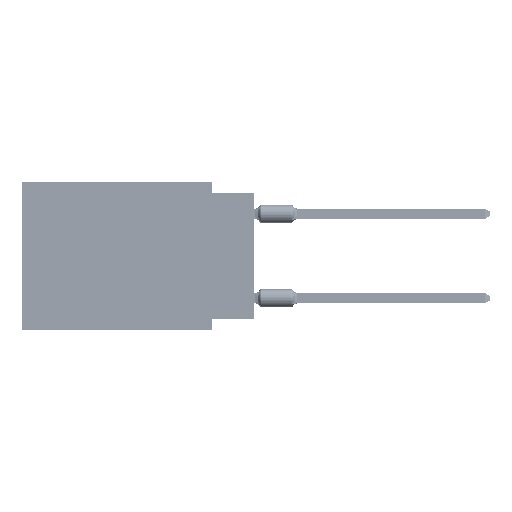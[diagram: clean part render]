
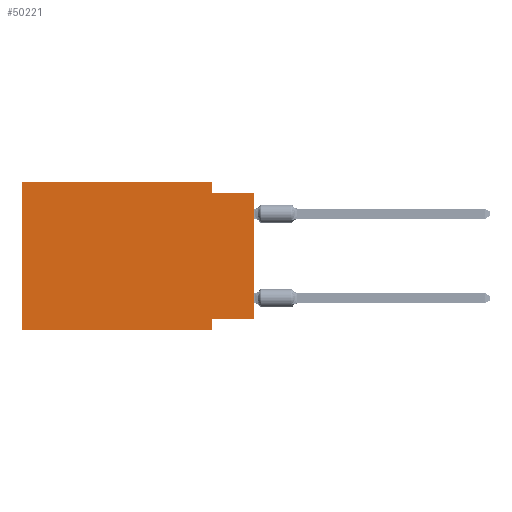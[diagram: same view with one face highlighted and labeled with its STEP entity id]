
A CAD part, left-side view. The second image highlights one B-rep face of the part: STEP entity #50221.
In plain terms, the highlighted planar face has unit normal (-1, 0, 0).
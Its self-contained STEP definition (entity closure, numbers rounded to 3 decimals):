
#461 = EDGE_CURVE ( 'NONE', #86852, #19791, #19772, .T. ) ;
#922 = VECTOR ( 'NONE', #32858, 1000. ) ;
#1708 = VECTOR ( 'NONE', #90868, 1000. ) ;
#1770 = CARTESIAN_POINT ( 'NONE',  ( 0., 13.97, 0. ) ) ;
#2707 = DIRECTION ( 'NONE',  ( 0., 0., 1. ) ) ;
#5888 = EDGE_CURVE ( 'NONE', #55395, #71463, #52211, .T. ) ;
#8643 = ORIENTED_EDGE ( 'NONE', *, *, #45282, .T. ) ;
#9731 = CARTESIAN_POINT ( 'NONE',  ( 0., 2.54, -8.255 ) ) ;
#12291 = VECTOR ( 'NONE', #2707, 1000. ) ;
#13193 = CARTESIAN_POINT ( 'NONE',  ( 0., 2.54, -0.635 ) ) ;
#16530 = VERTEX_POINT ( 'NONE', #30791 ) ;
#16608 = CARTESIAN_POINT ( 'NONE',  ( 0., 0., 0. ) ) ;
#19772 = LINE ( 'NONE', #77205, #922 ) ;
#19791 = VERTEX_POINT ( 'NONE', #26184 ) ;
#19880 = CARTESIAN_POINT ( 'NONE',  ( 0., 2.54, 0. ) ) ;
#20697 = LINE ( 'NONE', #43556, #22331 ) ;
#21333 = CARTESIAN_POINT ( 'NONE',  ( 0., 2.54, -8.89 ) ) ;
#21798 = LINE ( 'NONE', #21333, #37331 ) ;
#22331 = VECTOR ( 'NONE', #70205, 1000. ) ;
#22988 = ORIENTED_EDGE ( 'NONE', *, *, #48648, .F. ) ;
#24152 = CARTESIAN_POINT ( 'NONE',  ( 0., 0., -8.255 ) ) ;
#26184 = CARTESIAN_POINT ( 'NONE',  ( 0., 0., -0.635 ) ) ;
#30791 = CARTESIAN_POINT ( 'NONE',  ( 0., 0., -8.255 ) ) ;
#31715 = ORIENTED_EDGE ( 'NONE', *, *, #51398, .F. ) ;
#32858 = DIRECTION ( 'NONE',  ( 0., -1., 0. ) ) ;
#33879 = DIRECTION ( 'NONE',  ( 1., 0., 0. ) ) ;
#35646 = ORIENTED_EDGE ( 'NONE', *, *, #461, .F. ) ;
#37331 = VECTOR ( 'NONE', #62912, 1000. ) ;
#37951 = ORIENTED_EDGE ( 'NONE', *, *, #57464, .T. ) ;
#39762 = ORIENTED_EDGE ( 'NONE', *, *, #5888, .F. ) ;
#40905 = PLANE ( 'NONE',  #61109 ) ;
#43556 = CARTESIAN_POINT ( 'NONE',  ( 0., 13.97, -8.89 ) ) ;
#45282 = EDGE_CURVE ( 'NONE', #16530, #19791, #86662, .T. ) ;
#45919 = CARTESIAN_POINT ( 'NONE',  ( 0., 2.54, 0. ) ) ;
#47724 = VECTOR ( 'NONE', #58746, 1000. ) ;
#47904 = FACE_OUTER_BOUND ( 'NONE', #61583, .T. ) ;
#48648 = EDGE_CURVE ( 'NONE', #71359, #90215, #21798, .T. ) ;
#50221 = ADVANCED_FACE ( 'NONE', ( #47904 ), #40905, .F. ) ;
#51398 = EDGE_CURVE ( 'NONE', #88895, #86852, #89941, .T. ) ;
#52211 = LINE ( 'NONE', #86785, #12291 ) ;
#55395 = VERTEX_POINT ( 'NONE', #70302 ) ;
#57464 = EDGE_CURVE ( 'NONE', #55395, #90215, #20697, .T. ) ;
#58125 = EDGE_CURVE ( 'NONE', #16530, #71359, #73648, .T. ) ;
#58746 = DIRECTION ( 'NONE',  ( 0., -1., 0. ) ) ;
#59101 = DIRECTION ( 'NONE',  ( 0., 0., 1. ) ) ;
#59652 = VECTOR ( 'NONE', #81095, 1000. ) ;
#61109 = AXIS2_PLACEMENT_3D ( 'NONE', #69363, #33879, #90853 ) ;
#61583 = EDGE_LOOP ( 'NONE', ( #8643, #35646, #31715, #78894, #39762, #37951, #22988, #87907 ) ) ;
#62020 = VECTOR ( 'NONE', #59101, 1000. ) ;
#62912 = DIRECTION ( 'NONE',  ( 0., 0., -1. ) ) ;
#63377 = CARTESIAN_POINT ( 'NONE',  ( 0., 13.97, 0. ) ) ;
#66674 = LINE ( 'NONE', #1770, #47724 ) ;
#69363 = CARTESIAN_POINT ( 'NONE',  ( 0., 13.97, 0. ) ) ;
#70205 = DIRECTION ( 'NONE',  ( 0., -1., 0. ) ) ;
#70302 = CARTESIAN_POINT ( 'NONE',  ( 0., 13.97, -8.89 ) ) ;
#71359 = VERTEX_POINT ( 'NONE', #9731 ) ;
#71463 = VERTEX_POINT ( 'NONE', #63377 ) ;
#73648 = LINE ( 'NONE', #24152, #59652 ) ;
#77205 = CARTESIAN_POINT ( 'NONE',  ( 0., 0., -0.635 ) ) ;
#78894 = ORIENTED_EDGE ( 'NONE', *, *, #84627, .F. ) ;
#81095 = DIRECTION ( 'NONE',  ( 0., 1., 0. ) ) ;
#83747 = CARTESIAN_POINT ( 'NONE',  ( 0., 2.54, -8.89 ) ) ;
#84627 = EDGE_CURVE ( 'NONE', #71463, #88895, #66674, .T. ) ;
#86662 = LINE ( 'NONE', #16608, #62020 ) ;
#86785 = CARTESIAN_POINT ( 'NONE',  ( 0., 13.97, 0. ) ) ;
#86852 = VERTEX_POINT ( 'NONE', #13193 ) ;
#87907 = ORIENTED_EDGE ( 'NONE', *, *, #58125, .F. ) ;
#88895 = VERTEX_POINT ( 'NONE', #45919 ) ;
#89941 = LINE ( 'NONE', #19880, #1708 ) ;
#90215 = VERTEX_POINT ( 'NONE', #83747 ) ;
#90853 = DIRECTION ( 'NONE',  ( 0., 0., -1. ) ) ;
#90868 = DIRECTION ( 'NONE',  ( 0., 0., -1. ) ) ;
